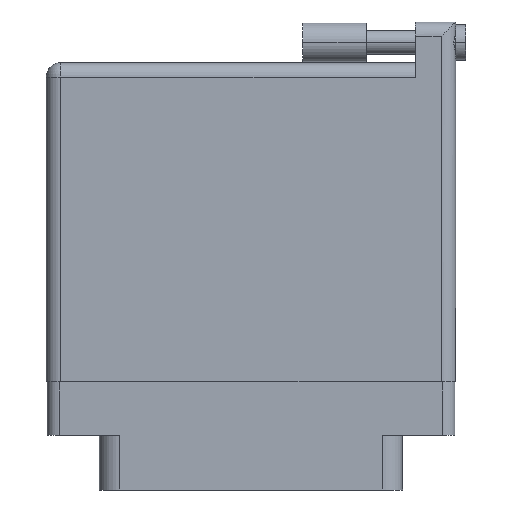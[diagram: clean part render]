
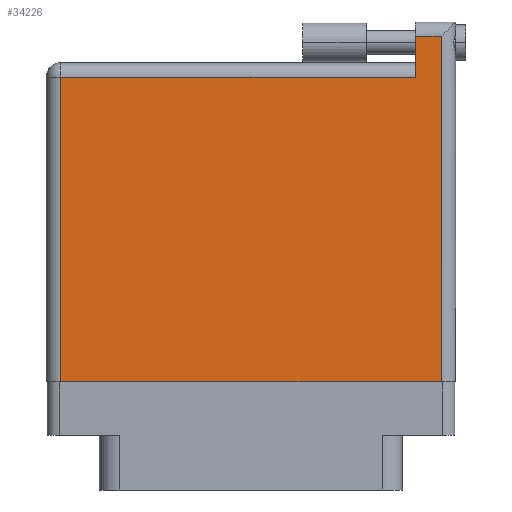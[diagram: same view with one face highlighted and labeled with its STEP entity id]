
A CAD part, front view. The second image highlights one B-rep face of the part: STEP entity #34226.
In plain terms, the highlighted face is planar.
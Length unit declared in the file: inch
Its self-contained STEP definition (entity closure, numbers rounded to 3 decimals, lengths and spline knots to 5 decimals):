
#1017 = CARTESIAN_POINT ( 'NONE',  ( 1.811, 1.696, 0. ) ) ;
#1494 = DIRECTION ( 'NONE',  ( 0., 0., -1. ) ) ;
#4737 = ORIENTED_EDGE ( 'NONE', *, *, #21883, .T. ) ;
#6822 = CARTESIAN_POINT ( 'NONE',  ( 0., 1.566, 0. ) ) ;
#6912 = LINE ( 'NONE', #13308, #23292 ) ;
#7212 = CARTESIAN_POINT ( 'NONE',  ( 1.811, 1.766, 0. ) ) ;
#7303 = DIRECTION ( 'NONE',  ( -1., 0., 0. ) ) ;
#7562 = FACE_OUTER_BOUND ( 'NONE', #23087, .T. ) ;
#7820 = DIRECTION ( 'NONE',  ( -1., 0., 0. ) ) ;
#8566 = EDGE_CURVE ( 'NONE', #30059, #21121, #32356, .T. ) ;
#10315 = EDGE_CURVE ( 'NONE', #16876, #14951, #15679, .T. ) ;
#10673 = EDGE_CURVE ( 'NONE', #21121, #16876, #21527, .T. ) ;
#10939 = ORIENTED_EDGE ( 'NONE', *, *, #10673, .T. ) ;
#11116 = EDGE_CURVE ( 'NONE', #20930, #30059, #17323, .T. ) ;
#11923 = CARTESIAN_POINT ( 'NONE',  ( 0.07, 0., 0. ) ) ;
#12279 = ORIENTED_EDGE ( 'NONE', *, *, #10315, .T. ) ;
#13308 = CARTESIAN_POINT ( 'NONE',  ( 0., 0., 0. ) ) ;
#14305 = CARTESIAN_POINT ( 'NONE',  ( 1.938, 1.696, 0. ) ) ;
#14646 = VERTEX_POINT ( 'NONE', #11923 ) ;
#14819 = EDGE_CURVE ( 'NONE', #14646, #20930, #6912, .T. ) ;
#14951 = VERTEX_POINT ( 'NONE', #15050 ) ;
#15050 = CARTESIAN_POINT ( 'NONE',  ( 0.07, 1.496, 0. ) ) ;
#15679 = LINE ( 'NONE', #26979, #23973 ) ;
#16379 = LINE ( 'NONE', #30922, #34848 ) ;
#16876 = VERTEX_POINT ( 'NONE', #18915 ) ;
#16918 = DIRECTION ( 'NONE',  ( 0., 1., 0. ) ) ;
#17323 = LINE ( 'NONE', #21947, #21907 ) ;
#17805 = PLANE ( 'NONE',  #24068 ) ;
#18915 = CARTESIAN_POINT ( 'NONE',  ( 1.811, 1.496, 0. ) ) ;
#20930 = VERTEX_POINT ( 'NONE', #28064 ) ;
#21121 = VERTEX_POINT ( 'NONE', #1017 ) ;
#21527 = LINE ( 'NONE', #7212, #31262 ) ;
#21883 = EDGE_CURVE ( 'NONE', #14951, #14646, #16379, .T. ) ;
#21907 = VECTOR ( 'NONE', #16918, 39.37008 ) ;
#21947 = CARTESIAN_POINT ( 'NONE',  ( 1.938, 1.766, 0. ) ) ;
#23087 = EDGE_LOOP ( 'NONE', ( #31714, #33110, #32090, #10939, #12279, #4737 ) ) ;
#23183 = CARTESIAN_POINT ( 'NONE',  ( 0., 1.696, 0. ) ) ;
#23292 = VECTOR ( 'NONE', #31880, 39.37008 ) ;
#23973 = VECTOR ( 'NONE', #7820, 39.37008 ) ;
#24068 = AXIS2_PLACEMENT_3D ( 'NONE', #6822, #1494, #25274 ) ;
#25274 = DIRECTION ( 'NONE',  ( -1., 0., 0. ) ) ;
#26979 = CARTESIAN_POINT ( 'NONE',  ( 0., 1.496, 0. ) ) ;
#28064 = CARTESIAN_POINT ( 'NONE',  ( 1.938, 0., 0. ) ) ;
#30059 = VERTEX_POINT ( 'NONE', #14305 ) ;
#30257 = VECTOR ( 'NONE', #7303, 39.37008 ) ;
#30922 = CARTESIAN_POINT ( 'NONE',  ( 0.07, 0., 0. ) ) ;
#31262 = VECTOR ( 'NONE', #34034, 39.37008 ) ;
#31714 = ORIENTED_EDGE ( 'NONE', *, *, #14819, .T. ) ;
#31880 = DIRECTION ( 'NONE',  ( 1., 0., 0. ) ) ;
#32090 = ORIENTED_EDGE ( 'NONE', *, *, #8566, .T. ) ;
#32356 = LINE ( 'NONE', #23183, #30257 ) ;
#33110 = ORIENTED_EDGE ( 'NONE', *, *, #11116, .T. ) ;
#33932 = DIRECTION ( 'NONE',  ( 0., -1., 0. ) ) ;
#34034 = DIRECTION ( 'NONE',  ( 0., -1., 0. ) ) ;
#34226 = ADVANCED_FACE ( 'NONE', ( #7562 ), #17805, .F. ) ;
#34848 = VECTOR ( 'NONE', #33932, 39.37008 ) ;
